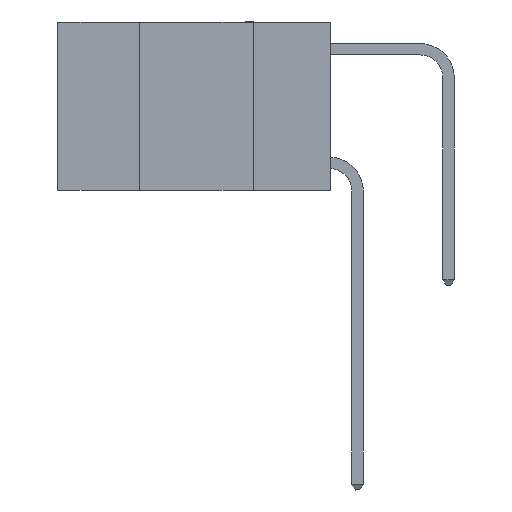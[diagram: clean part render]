
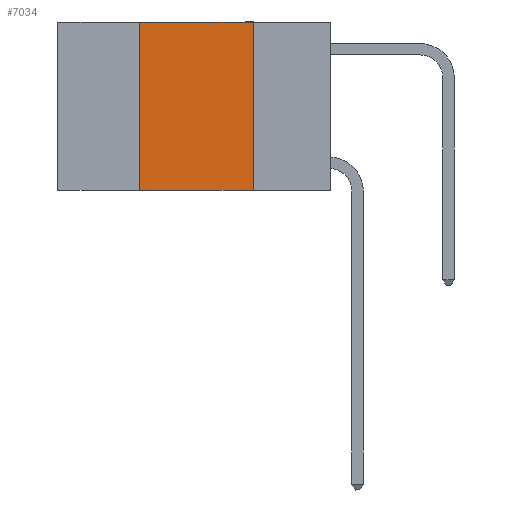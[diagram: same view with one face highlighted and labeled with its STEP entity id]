
A CAD part, left-side view. The second image highlights one B-rep face of the part: STEP entity #7034.
In plain terms, the highlighted planar face has unit normal (-1, 0, 0).
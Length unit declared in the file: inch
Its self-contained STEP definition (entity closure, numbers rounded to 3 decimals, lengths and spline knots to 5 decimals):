
#2546 = LINE ( 'NONE', #17821, #23049 ) ;
#2842 = CARTESIAN_POINT ( 'NONE',  ( 0., 0.6, -0.37 ) ) ;
#4639 = CARTESIAN_POINT ( 'NONE',  ( 0., 0.17, -0.37 ) ) ;
#4865 = FACE_OUTER_BOUND ( 'NONE', #8245, .T. ) ;
#7034 = ADVANCED_FACE ( 'NONE', ( #4865 ), #20933, .F. ) ;
#7328 = DIRECTION ( 'NONE',  ( 0., -1., 0. ) ) ;
#7857 = CARTESIAN_POINT ( 'NONE',  ( 0., 0.6, 0. ) ) ;
#8174 = EDGE_CURVE ( 'NONE', #10714, #27525, #21904, .T. ) ;
#8245 = EDGE_LOOP ( 'NONE', ( #24425, #18589, #12815, #12111 ) ) ;
#9244 = VERTEX_POINT ( 'NONE', #26006 ) ;
#9514 = CARTESIAN_POINT ( 'NONE',  ( 0., 0.6, 0. ) ) ;
#10087 = DIRECTION ( 'NONE',  ( 1., 0., 0. ) ) ;
#10714 = VERTEX_POINT ( 'NONE', #16894 ) ;
#10781 = CARTESIAN_POINT ( 'NONE',  ( 0., 0.42, 0. ) ) ;
#11065 = CARTESIAN_POINT ( 'NONE',  ( 0., 0.42, 0. ) ) ;
#11341 = DIRECTION ( 'NONE',  ( 0., 0., -1. ) ) ;
#11683 = EDGE_CURVE ( 'NONE', #27468, #9244, #13827, .T. ) ;
#11687 = DIRECTION ( 'NONE',  ( 0., -1., 0. ) ) ;
#11790 = LINE ( 'NONE', #10781, #16231 ) ;
#12111 = ORIENTED_EDGE ( 'NONE', *, *, #8174, .T. ) ;
#12815 = ORIENTED_EDGE ( 'NONE', *, *, #24694, .F. ) ;
#13540 = VECTOR ( 'NONE', #11687, 39.37008 ) ;
#13827 = LINE ( 'NONE', #9514, #13540 ) ;
#15177 = DIRECTION ( 'NONE',  ( 0., 0., 1. ) ) ;
#15440 = VECTOR ( 'NONE', #7328, 39.37008 ) ;
#16231 = VECTOR ( 'NONE', #15177, 39.37008 ) ;
#16894 = CARTESIAN_POINT ( 'NONE',  ( 0., 0.42, -0.37 ) ) ;
#17821 = CARTESIAN_POINT ( 'NONE',  ( 0., 0.17, 0. ) ) ;
#18589 = ORIENTED_EDGE ( 'NONE', *, *, #11683, .F. ) ;
#20933 = PLANE ( 'NONE',  #26236 ) ;
#21904 = LINE ( 'NONE', #2842, #15440 ) ;
#23049 = VECTOR ( 'NONE', #11341, 39.37008 ) ;
#24425 = ORIENTED_EDGE ( 'NONE', *, *, #24855, .F. ) ;
#24694 = EDGE_CURVE ( 'NONE', #10714, #27468, #11790, .T. ) ;
#24855 = EDGE_CURVE ( 'NONE', #9244, #27525, #2546, .T. ) ;
#25331 = DIRECTION ( 'NONE',  ( 0., 0., -1. ) ) ;
#26006 = CARTESIAN_POINT ( 'NONE',  ( 0., 0.17, 0. ) ) ;
#26236 = AXIS2_PLACEMENT_3D ( 'NONE', #7857, #10087, #25331 ) ;
#27468 = VERTEX_POINT ( 'NONE', #11065 ) ;
#27525 = VERTEX_POINT ( 'NONE', #4639 ) ;
